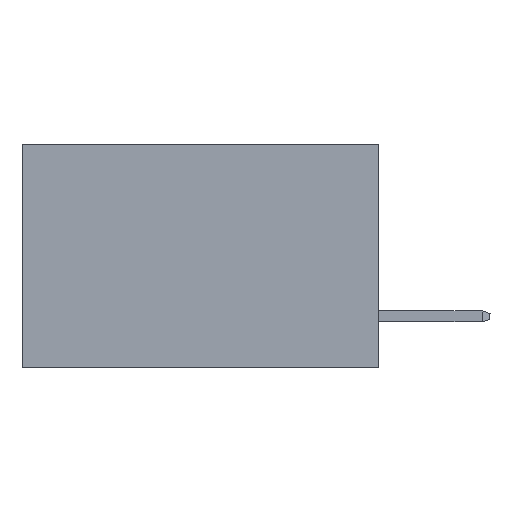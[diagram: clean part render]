
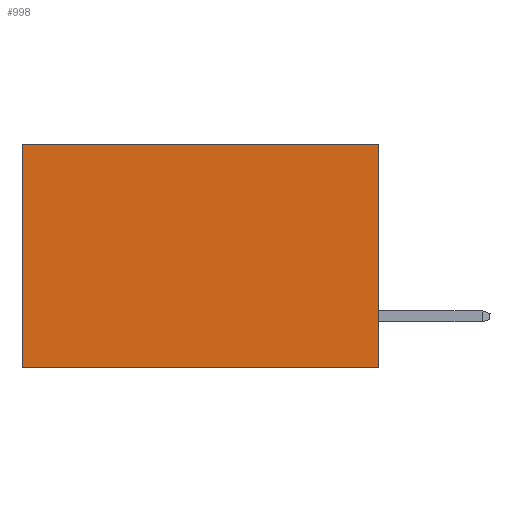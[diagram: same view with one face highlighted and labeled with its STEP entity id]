
A CAD part, left-side view. The second image highlights one B-rep face of the part: STEP entity #998.
In plain terms, the highlighted planar face has unit normal (-1, 0, 0).
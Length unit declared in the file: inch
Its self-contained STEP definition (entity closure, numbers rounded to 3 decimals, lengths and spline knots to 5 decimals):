
#318 = LINE ( 'NONE', #14605, #11641 ) ;
#998 = ADVANCED_FACE ( 'NONE', ( #14195 ), #3708, .F. ) ;
#2310 = DIRECTION ( 'NONE',  ( 0., 0., -1. ) ) ;
#2409 = DIRECTION ( 'NONE',  ( 1., 0., 0. ) ) ;
#2711 = EDGE_CURVE ( 'NONE', #5982, #6785, #11734, .T. ) ;
#2774 = CARTESIAN_POINT ( 'NONE',  ( 0.277, 0., 0. ) ) ;
#3708 = PLANE ( 'NONE',  #17740 ) ;
#5090 = EDGE_CURVE ( 'NONE', #7626, #5982, #22858, .T. ) ;
#5459 = VECTOR ( 'NONE', #2310, 39.37008 ) ;
#5982 = VERTEX_POINT ( 'NONE', #26108 ) ;
#6071 = CARTESIAN_POINT ( 'NONE',  ( 0.277, 0.59, 0. ) ) ;
#6203 = VECTOR ( 'NONE', #16770, 39.37008 ) ;
#6519 = DIRECTION ( 'NONE',  ( 0., 0., -1. ) ) ;
#6785 = VERTEX_POINT ( 'NONE', #14824 ) ;
#7626 = VERTEX_POINT ( 'NONE', #2774 ) ;
#10471 = CARTESIAN_POINT ( 'NONE',  ( 0.277, 0., -0.37 ) ) ;
#10781 = CARTESIAN_POINT ( 'NONE',  ( 0.277, 0.59, -0.37 ) ) ;
#11613 = VECTOR ( 'NONE', #14520, 39.37008 ) ;
#11641 = VECTOR ( 'NONE', #16749, 39.37008 ) ;
#11665 = LINE ( 'NONE', #10781, #5459 ) ;
#11734 = LINE ( 'NONE', #10471, #6203 ) ;
#12711 = VERTEX_POINT ( 'NONE', #6071 ) ;
#13572 = ORIENTED_EDGE ( 'NONE', *, *, #2711, .F. ) ;
#14195 = FACE_OUTER_BOUND ( 'NONE', #15876, .T. ) ;
#14262 = ORIENTED_EDGE ( 'NONE', *, *, #5090, .F. ) ;
#14520 = DIRECTION ( 'NONE',  ( 0., 0., -1. ) ) ;
#14605 = CARTESIAN_POINT ( 'NONE',  ( 0.277, 0., 0. ) ) ;
#14642 = CARTESIAN_POINT ( 'NONE',  ( 0.277, 0., -0.37 ) ) ;
#14824 = CARTESIAN_POINT ( 'NONE',  ( 0.277, 0.59, -0.37 ) ) ;
#15876 = EDGE_LOOP ( 'NONE', ( #24137, #13572, #14262, #25399 ) ) ;
#16749 = DIRECTION ( 'NONE',  ( 0., 1., 0. ) ) ;
#16770 = DIRECTION ( 'NONE',  ( 0., 1., 0. ) ) ;
#17740 = AXIS2_PLACEMENT_3D ( 'NONE', #26990, #2409, #6519 ) ;
#19793 = EDGE_CURVE ( 'NONE', #12711, #6785, #11665, .T. ) ;
#20323 = EDGE_CURVE ( 'NONE', #7626, #12711, #318, .T. ) ;
#22858 = LINE ( 'NONE', #14642, #11613 ) ;
#24137 = ORIENTED_EDGE ( 'NONE', *, *, #19793, .T. ) ;
#25399 = ORIENTED_EDGE ( 'NONE', *, *, #20323, .T. ) ;
#26108 = CARTESIAN_POINT ( 'NONE',  ( 0.277, 0., -0.37 ) ) ;
#26990 = CARTESIAN_POINT ( 'NONE',  ( 0.277, 0., -0.37 ) ) ;
